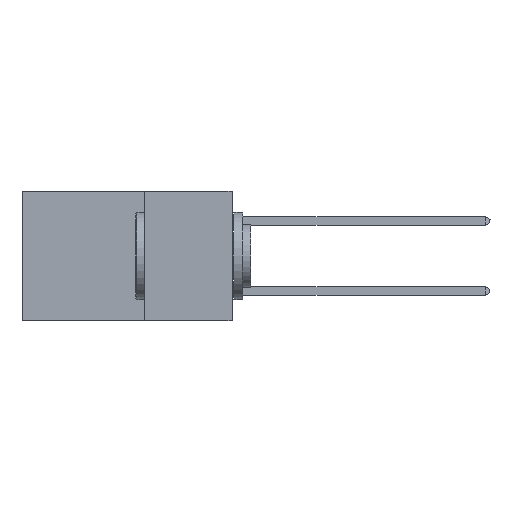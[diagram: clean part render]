
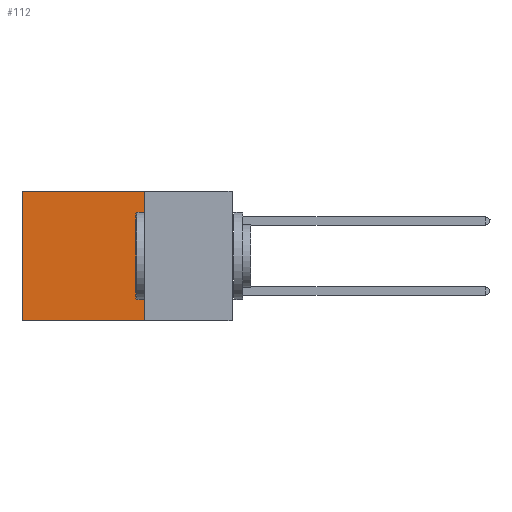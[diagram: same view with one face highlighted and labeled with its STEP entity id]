
A CAD part, left-side view. The second image highlights one B-rep face of the part: STEP entity #112.
In plain terms, the highlighted planar face has unit normal (-1, 0, 0).
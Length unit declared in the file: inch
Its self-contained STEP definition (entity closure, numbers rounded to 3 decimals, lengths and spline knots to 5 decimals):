
#112 = ADVANCED_FACE ( 'NONE', ( #18065 ), #11897, .F. ) ;
#3230 = ORIENTED_EDGE ( 'NONE', *, *, #6589, .F. ) ;
#5104 = VECTOR ( 'NONE', #40327, 39.37008 ) ;
#5627 = AXIS2_PLACEMENT_3D ( 'NONE', #8463, #12048, #36919 ) ;
#5779 = CARTESIAN_POINT ( 'NONE',  ( 0.2875, 0.6, 0. ) ) ;
#6589 = EDGE_CURVE ( 'NONE', #12086, #15691, #20978, .T. ) ;
#6699 = DIRECTION ( 'NONE',  ( 0., 1., 0. ) ) ;
#7817 = LINE ( 'NONE', #24516, #10088 ) ;
#8161 = VERTEX_POINT ( 'NONE', #5779 ) ;
#8325 = EDGE_CURVE ( 'NONE', #12086, #8161, #7817, .T. ) ;
#8463 = CARTESIAN_POINT ( 'NONE',  ( 0.2875, 0.25, 0. ) ) ;
#8640 = ORIENTED_EDGE ( 'NONE', *, *, #8325, .T. ) ;
#9410 = CARTESIAN_POINT ( 'NONE',  ( 0.2875, 0.6, -0.37 ) ) ;
#10088 = VECTOR ( 'NONE', #6699, 39.37008 ) ;
#11897 = PLANE ( 'NONE',  #5627 ) ;
#12048 = DIRECTION ( 'NONE',  ( 1., 0., 0. ) ) ;
#12086 = VERTEX_POINT ( 'NONE', #39350 ) ;
#15691 = VERTEX_POINT ( 'NONE', #40672 ) ;
#16321 = EDGE_CURVE ( 'NONE', #15691, #28312, #25144, .T. ) ;
#16597 = ORIENTED_EDGE ( 'NONE', *, *, #16321, .F. ) ;
#18065 = FACE_OUTER_BOUND ( 'NONE', #33600, .T. ) ;
#18961 = DIRECTION ( 'NONE',  ( 0., 0., -1. ) ) ;
#19201 = CARTESIAN_POINT ( 'NONE',  ( 0.2875, 0.25, -0.37 ) ) ;
#19878 = VECTOR ( 'NONE', #18961, 39.37008 ) ;
#20978 = LINE ( 'NONE', #40099, #19878 ) ;
#24516 = CARTESIAN_POINT ( 'NONE',  ( 0.2875, 0.25, 0. ) ) ;
#25144 = LINE ( 'NONE', #19201, #33428 ) ;
#26161 = CARTESIAN_POINT ( 'NONE',  ( 0.2875, 0.6, 0. ) ) ;
#28312 = VERTEX_POINT ( 'NONE', #9410 ) ;
#33259 = DIRECTION ( 'NONE',  ( 0., 1., 0. ) ) ;
#33428 = VECTOR ( 'NONE', #33259, 39.37008 ) ;
#33510 = LINE ( 'NONE', #26161, #5104 ) ;
#33600 = EDGE_LOOP ( 'NONE', ( #37864, #16597, #3230, #8640 ) ) ;
#36919 = DIRECTION ( 'NONE',  ( 0., 0., -1. ) ) ;
#37864 = ORIENTED_EDGE ( 'NONE', *, *, #44122, .T. ) ;
#39350 = CARTESIAN_POINT ( 'NONE',  ( 0.2875, 0.25, 0. ) ) ;
#40099 = CARTESIAN_POINT ( 'NONE',  ( 0.2875, 0.25, 0. ) ) ;
#40327 = DIRECTION ( 'NONE',  ( 0., 0., -1. ) ) ;
#40672 = CARTESIAN_POINT ( 'NONE',  ( 0.2875, 0.25, -0.37 ) ) ;
#44122 = EDGE_CURVE ( 'NONE', #8161, #28312, #33510, .T. ) ;
